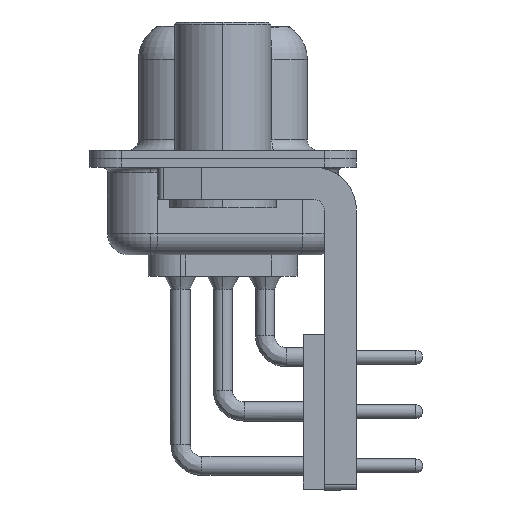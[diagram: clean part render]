
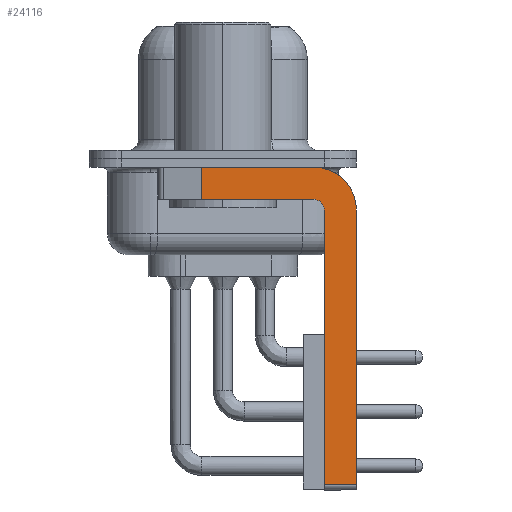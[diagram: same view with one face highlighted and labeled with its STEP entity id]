
A CAD part, left-side view. The second image highlights one B-rep face of the part: STEP entity #24116.
In plain terms, the highlighted planar face has unit normal (-1, 0, 0).
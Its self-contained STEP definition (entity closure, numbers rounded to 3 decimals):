
#167 = LINE ( 'NONE', #23580, #16670 ) ;
#513 = CARTESIAN_POINT ( 'NONE',  ( -2.9, -4.25, -1.9 ) ) ;
#1290 = FACE_OUTER_BOUND ( 'NONE', #3047, .T. ) ;
#1455 = ORIENTED_EDGE ( 'NONE', *, *, #26907, .F. ) ;
#1510 = DIRECTION ( 'NONE',  ( 1., 0., 0. ) ) ;
#1591 = LINE ( 'NONE', #513, #5985 ) ;
#2617 = VECTOR ( 'NONE', #3454, 1000. ) ;
#2946 = LINE ( 'NONE', #7841, #13036 ) ;
#3025 = CARTESIAN_POINT ( 'NONE',  ( -2.9, 0.978, -0.4 ) ) ;
#3047 = EDGE_LOOP ( 'NONE', ( #1455, #23514, #17581, #16416, #14943, #21278, #23551, #13727 ) ) ;
#3296 = LINE ( 'NONE', #9862, #2617 ) ;
#3454 = DIRECTION ( 'NONE',  ( 0., 0., -1. ) ) ;
#3671 = VERTEX_POINT ( 'NONE', #20987 ) ;
#4200 = VERTEX_POINT ( 'NONE', #9184 ) ;
#4372 = CARTESIAN_POINT ( 'NONE',  ( -2.9, -6.25, -2.4 ) ) ;
#5135 = AXIS2_PLACEMENT_3D ( 'NONE', #23376, #10477, #25606 ) ;
#5336 = CARTESIAN_POINT ( 'NONE',  ( -2.9, -4.25, -1.9 ) ) ;
#5528 = LINE ( 'NONE', #11512, #13253 ) ;
#5985 = VECTOR ( 'NONE', #13388, 1000. ) ;
#7581 = LINE ( 'NONE', #22483, #18353 ) ;
#7728 = DIRECTION ( 'NONE',  ( 1., 0., 0. ) ) ;
#7812 = CARTESIAN_POINT ( 'NONE',  ( -2.9, -4.25, -2.4 ) ) ;
#7841 = CARTESIAN_POINT ( 'NONE',  ( -2.9, 0.978, -1.9 ) ) ;
#8018 = CIRCLE ( 'NONE', #5135, 0.5 ) ;
#8241 = VERTEX_POINT ( 'NONE', #3025 ) ;
#8898 = VERTEX_POINT ( 'NONE', #22727 ) ;
#9184 = CARTESIAN_POINT ( 'NONE',  ( -2.9, -6.25, -15.25 ) ) ;
#9862 = CARTESIAN_POINT ( 'NONE',  ( -2.9, -6.25, -2.4 ) ) ;
#10011 = DIRECTION ( 'NONE',  ( 0., 0., -1. ) ) ;
#10477 = DIRECTION ( 'NONE',  ( -1., 0., 0. ) ) ;
#11286 = AXIS2_PLACEMENT_3D ( 'NONE', #7812, #1510, #16536 ) ;
#11311 = EDGE_CURVE ( 'NONE', #8241, #19359, #2946, .T. ) ;
#11512 = CARTESIAN_POINT ( 'NONE',  ( -2.9, -4.25, -15.25 ) ) ;
#12789 = EDGE_CURVE ( 'NONE', #21286, #19359, #1591, .T. ) ;
#13036 = VECTOR ( 'NONE', #10011, 1000. ) ;
#13253 = VECTOR ( 'NONE', #15748, 1000. ) ;
#13388 = DIRECTION ( 'NONE',  ( 0., 1., 0. ) ) ;
#13689 = EDGE_CURVE ( 'NONE', #3671, #20434, #26514, .T. ) ;
#13727 = ORIENTED_EDGE ( 'NONE', *, *, #13689, .F. ) ;
#14389 = PLANE ( 'NONE',  #11286 ) ;
#14943 = ORIENTED_EDGE ( 'NONE', *, *, #17685, .F. ) ;
#15748 = DIRECTION ( 'NONE',  ( 0., -1., 0. ) ) ;
#16015 = EDGE_CURVE ( 'NONE', #8898, #21286, #8018, .T. ) ;
#16224 = CARTESIAN_POINT ( 'NONE',  ( -2.9, -4.75, -15.25 ) ) ;
#16416 = ORIENTED_EDGE ( 'NONE', *, *, #16015, .F. ) ;
#16536 = DIRECTION ( 'NONE',  ( 0., 0., -1. ) ) ;
#16670 = VECTOR ( 'NONE', #17076, 1000. ) ;
#17013 = VERTEX_POINT ( 'NONE', #16224 ) ;
#17076 = DIRECTION ( 'NONE',  ( 0., 0., 1. ) ) ;
#17581 = ORIENTED_EDGE ( 'NONE', *, *, #12789, .F. ) ;
#17685 = EDGE_CURVE ( 'NONE', #17013, #8898, #167, .T. ) ;
#18353 = VECTOR ( 'NONE', #24692, 1000. ) ;
#18897 = AXIS2_PLACEMENT_3D ( 'NONE', #20639, #7728, #22775 ) ;
#19359 = VERTEX_POINT ( 'NONE', #25343 ) ;
#20434 = VERTEX_POINT ( 'NONE', #4372 ) ;
#20639 = CARTESIAN_POINT ( 'NONE',  ( -2.9, -4.25, -2.4 ) ) ;
#20987 = CARTESIAN_POINT ( 'NONE',  ( -2.9, -4.25, -0.4 ) ) ;
#21278 = ORIENTED_EDGE ( 'NONE', *, *, #27495, .T. ) ;
#21286 = VERTEX_POINT ( 'NONE', #5336 ) ;
#22483 = CARTESIAN_POINT ( 'NONE',  ( -2.9, 3., -0.4 ) ) ;
#22727 = CARTESIAN_POINT ( 'NONE',  ( -2.9, -4.75, -2.4 ) ) ;
#22775 = DIRECTION ( 'NONE',  ( 0., 0., -1. ) ) ;
#23376 = CARTESIAN_POINT ( 'NONE',  ( -2.9, -4.25, -2.4 ) ) ;
#23514 = ORIENTED_EDGE ( 'NONE', *, *, #11311, .T. ) ;
#23551 = ORIENTED_EDGE ( 'NONE', *, *, #24629, .F. ) ;
#23580 = CARTESIAN_POINT ( 'NONE',  ( -2.9, -4.75, -15.5 ) ) ;
#24116 = ADVANCED_FACE ( 'NONE', ( #1290 ), #14389, .F. ) ;
#24629 = EDGE_CURVE ( 'NONE', #20434, #4200, #3296, .T. ) ;
#24692 = DIRECTION ( 'NONE',  ( 0., -1., 0. ) ) ;
#25343 = CARTESIAN_POINT ( 'NONE',  ( -2.9, 0.978, -1.9 ) ) ;
#25606 = DIRECTION ( 'NONE',  ( 0., 0., 1. ) ) ;
#26514 = CIRCLE ( 'NONE', #18897, 2. ) ;
#26907 = EDGE_CURVE ( 'NONE', #8241, #3671, #7581, .T. ) ;
#27495 = EDGE_CURVE ( 'NONE', #17013, #4200, #5528, .T. ) ;
